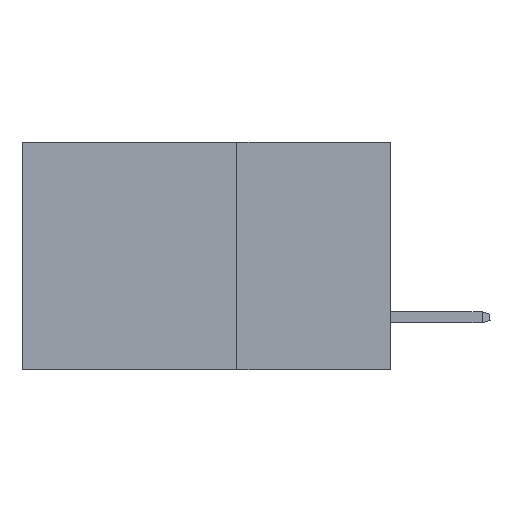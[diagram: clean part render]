
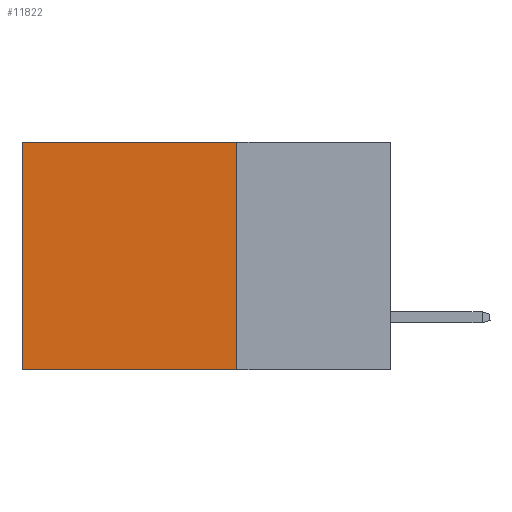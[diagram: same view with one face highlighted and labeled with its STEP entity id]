
A CAD part, left-side view. The second image highlights one B-rep face of the part: STEP entity #11822.
In plain terms, the highlighted planar face has unit normal (-1, 0, 0).
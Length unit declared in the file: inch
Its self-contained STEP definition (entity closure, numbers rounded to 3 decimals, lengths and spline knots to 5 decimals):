
#1245 = DIRECTION ( 'NONE',  ( 1., 0., 0. ) ) ;
#1519 = LINE ( 'NONE', #28517, #6799 ) ;
#1808 = EDGE_CURVE ( 'NONE', #11833, #30517, #18549, .T. ) ;
#3708 = VERTEX_POINT ( 'NONE', #8750 ) ;
#3976 = AXIS2_PLACEMENT_3D ( 'NONE', #34359, #1245, #22470 ) ;
#4236 = ORIENTED_EDGE ( 'NONE', *, *, #14147, .T. ) ;
#6799 = VECTOR ( 'NONE', #37504, 39.37008 ) ;
#8750 = CARTESIAN_POINT ( 'NONE',  ( 0.2875, 0.6, 0. ) ) ;
#9433 = VECTOR ( 'NONE', #20632, 39.37008 ) ;
#10139 = EDGE_CURVE ( 'NONE', #11833, #3708, #25465, .T. ) ;
#10292 = ORIENTED_EDGE ( 'NONE', *, *, #10139, .T. ) ;
#10354 = PLANE ( 'NONE',  #3976 ) ;
#10543 = CARTESIAN_POINT ( 'NONE',  ( 0.2875, 0.25, -0.37 ) ) ;
#11699 = CARTESIAN_POINT ( 'NONE',  ( 0.2875, 0.25, 0. ) ) ;
#11822 = ADVANCED_FACE ( 'NONE', ( #27745 ), #10354, .F. ) ;
#11833 = VERTEX_POINT ( 'NONE', #28508 ) ;
#14147 = EDGE_CURVE ( 'NONE', #3708, #37428, #1519, .T. ) ;
#14366 = LINE ( 'NONE', #10543, #37286 ) ;
#14762 = DIRECTION ( 'NONE',  ( 0., 0., -1. ) ) ;
#15360 = ORIENTED_EDGE ( 'NONE', *, *, #21134, .F. ) ;
#16670 = VECTOR ( 'NONE', #14762, 39.37008 ) ;
#18549 = LINE ( 'NONE', #11699, #16670 ) ;
#19822 = CARTESIAN_POINT ( 'NONE',  ( 0.2875, 0.6, -0.37 ) ) ;
#20632 = DIRECTION ( 'NONE',  ( 0., 1., 0. ) ) ;
#20996 = EDGE_LOOP ( 'NONE', ( #4236, #15360, #33854, #10292 ) ) ;
#21134 = EDGE_CURVE ( 'NONE', #30517, #37428, #14366, .T. ) ;
#22470 = DIRECTION ( 'NONE',  ( 0., 0., -1. ) ) ;
#25465 = LINE ( 'NONE', #38517, #9433 ) ;
#26872 = CARTESIAN_POINT ( 'NONE',  ( 0.2875, 0.25, -0.37 ) ) ;
#27745 = FACE_OUTER_BOUND ( 'NONE', #20996, .T. ) ;
#28508 = CARTESIAN_POINT ( 'NONE',  ( 0.2875, 0.25, 0. ) ) ;
#28517 = CARTESIAN_POINT ( 'NONE',  ( 0.2875, 0.6, 0. ) ) ;
#30517 = VERTEX_POINT ( 'NONE', #26872 ) ;
#33854 = ORIENTED_EDGE ( 'NONE', *, *, #1808, .F. ) ;
#34359 = CARTESIAN_POINT ( 'NONE',  ( 0.2875, 0.25, 0. ) ) ;
#37286 = VECTOR ( 'NONE', #37565, 39.37008 ) ;
#37428 = VERTEX_POINT ( 'NONE', #19822 ) ;
#37504 = DIRECTION ( 'NONE',  ( 0., 0., -1. ) ) ;
#37565 = DIRECTION ( 'NONE',  ( 0., 1., 0. ) ) ;
#38517 = CARTESIAN_POINT ( 'NONE',  ( 0.2875, 0.25, 0. ) ) ;
